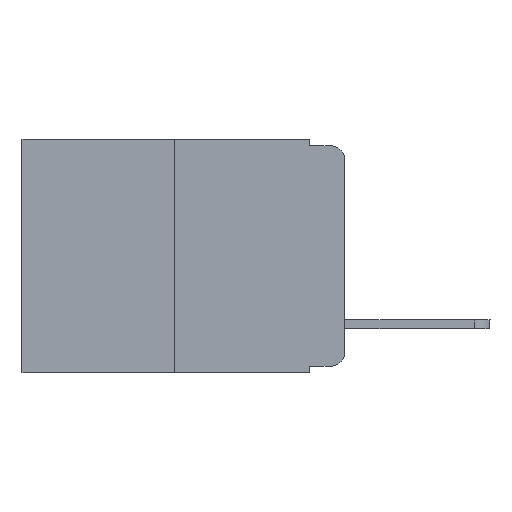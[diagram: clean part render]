
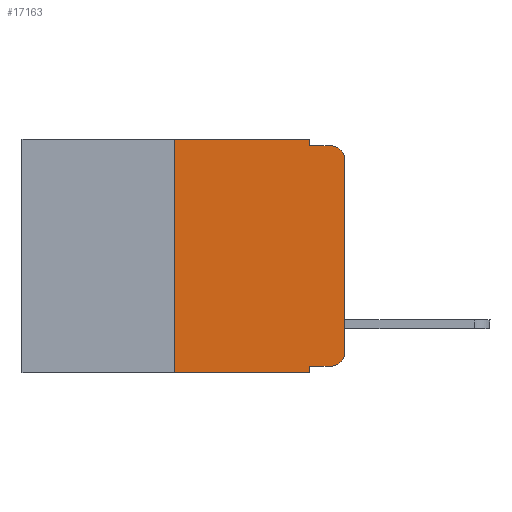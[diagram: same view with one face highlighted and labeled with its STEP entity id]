
A CAD part, left-side view. The second image highlights one B-rep face of the part: STEP entity #17163.
In plain terms, the highlighted planar face has unit normal (-1, 0, 0).
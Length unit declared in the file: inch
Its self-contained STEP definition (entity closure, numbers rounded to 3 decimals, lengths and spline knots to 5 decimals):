
#25 = CARTESIAN_POINT ( 'NONE',  ( 0., 0.473, 0. ) ) ;
#156 = LINE ( 'NONE', #4630, #2703 ) ;
#206 = EDGE_CURVE ( 'NONE', #1148, #16607, #7201, .T. ) ;
#306 = VECTOR ( 'NONE', #5939, 39.37008 ) ;
#526 = EDGE_CURVE ( 'NONE', #20060, #1148, #8143, .T. ) ;
#609 = LINE ( 'NONE', #7110, #16516 ) ;
#885 = EDGE_CURVE ( 'NONE', #12155, #20060, #12541, .T. ) ;
#1148 = VERTEX_POINT ( 'NONE', #8923 ) ;
#1955 = VECTOR ( 'NONE', #15496, 39.37008 ) ;
#2307 = CARTESIAN_POINT ( 'NONE',  ( 0., 0.02, -0.01 ) ) ;
#2349 = EDGE_CURVE ( 'NONE', #11535, #4945, #4373, .T. ) ;
#2442 = CARTESIAN_POINT ( 'NONE',  ( 0., 0.02, -0.333 ) ) ;
#2703 = VECTOR ( 'NONE', #9926, 39.37008 ) ;
#3430 = ORIENTED_EDGE ( 'NONE', *, *, #206, .T. ) ;
#3432 = DIRECTION ( 'NONE',  ( 0., 0., -1. ) ) ;
#3862 = CARTESIAN_POINT ( 'NONE',  ( 0., 0.473, -0.343 ) ) ;
#3900 = DIRECTION ( 'NONE',  ( 0., 0., -1. ) ) ;
#3972 = VERTEX_POINT ( 'NONE', #5733 ) ;
#4373 = LINE ( 'NONE', #19002, #14022 ) ;
#4630 = CARTESIAN_POINT ( 'NONE',  ( 0., 0.051, 0. ) ) ;
#4945 = VERTEX_POINT ( 'NONE', #18757 ) ;
#5733 = CARTESIAN_POINT ( 'NONE',  ( 0., 0.051, -0.01 ) ) ;
#5939 = DIRECTION ( 'NONE',  ( 0., -1., 0. ) ) ;
#6059 = VECTOR ( 'NONE', #16985, 39.37008 ) ;
#6770 = AXIS2_PLACEMENT_3D ( 'NONE', #25, #14555, #3432 ) ;
#7110 = CARTESIAN_POINT ( 'NONE',  ( 0., 0.473, 0. ) ) ;
#7201 = CIRCLE ( 'NONE', #10912, 0.02 ) ;
#7504 = CARTESIAN_POINT ( 'NONE',  ( 0., 0.051, 0. ) ) ;
#8056 = ORIENTED_EDGE ( 'NONE', *, *, #17466, .F. ) ;
#8143 = LINE ( 'NONE', #17993, #16339 ) ;
#8671 = ORIENTED_EDGE ( 'NONE', *, *, #885, .T. ) ;
#8803 = EDGE_CURVE ( 'NONE', #10711, #9276, #16306, .T. ) ;
#8923 = CARTESIAN_POINT ( 'NONE',  ( 0., 0., -0.03 ) ) ;
#8993 = ORIENTED_EDGE ( 'NONE', *, *, #526, .T. ) ;
#9030 = LINE ( 'NONE', #3862, #1955 ) ;
#9276 = VERTEX_POINT ( 'NONE', #16469 ) ;
#9844 = DIRECTION ( 'NONE',  ( 0., 0., -1. ) ) ;
#9926 = DIRECTION ( 'NONE',  ( 0., 0., -1. ) ) ;
#10392 = CARTESIAN_POINT ( 'NONE',  ( 0., 0.051, -0.333 ) ) ;
#10711 = VERTEX_POINT ( 'NONE', #15401 ) ;
#10912 = AXIS2_PLACEMENT_3D ( 'NONE', #11940, #11845, #3900 ) ;
#11369 = FACE_OUTER_BOUND ( 'NONE', #12561, .T. ) ;
#11535 = VERTEX_POINT ( 'NONE', #16652 ) ;
#11582 = PLANE ( 'NONE',  #6770 ) ;
#11619 = EDGE_CURVE ( 'NONE', #4945, #18305, #609, .T. ) ;
#11752 = ORIENTED_EDGE ( 'NONE', *, *, #2349, .F. ) ;
#11845 = DIRECTION ( 'NONE',  ( -1., 0., 0. ) ) ;
#11940 = CARTESIAN_POINT ( 'NONE',  ( 0., 0.02, -0.03 ) ) ;
#12155 = VERTEX_POINT ( 'NONE', #2442 ) ;
#12209 = LINE ( 'NONE', #10392, #6059 ) ;
#12312 = DIRECTION ( 'NONE',  ( 0., 0., 1. ) ) ;
#12541 = CIRCLE ( 'NONE', #16273, 0.02 ) ;
#12561 = EDGE_LOOP ( 'NONE', ( #8993, #3430, #8056, #15671, #16234, #11752, #13490, #19317, #12961, #8671 ) ) ;
#12621 = LINE ( 'NONE', #20562, #306 ) ;
#12871 = CARTESIAN_POINT ( 'NONE',  ( 0., 0., -0.313 ) ) ;
#12961 = ORIENTED_EDGE ( 'NONE', *, *, #17292, .T. ) ;
#13490 = ORIENTED_EDGE ( 'NONE', *, *, #16862, .T. ) ;
#13568 = DIRECTION ( 'NONE',  ( 0., -1., 0. ) ) ;
#14022 = VECTOR ( 'NONE', #12312, 39.37008 ) ;
#14555 = DIRECTION ( 'NONE',  ( 1., 0., 0. ) ) ;
#14594 = DIRECTION ( 'NONE',  ( 0., 0., 1. ) ) ;
#14604 = CARTESIAN_POINT ( 'NONE',  ( 0., 0.051, 0. ) ) ;
#15401 = CARTESIAN_POINT ( 'NONE',  ( 0., 0.051, -0.333 ) ) ;
#15496 = DIRECTION ( 'NONE',  ( 0., -1., 0. ) ) ;
#15671 = ORIENTED_EDGE ( 'NONE', *, *, #19745, .F. ) ;
#16234 = ORIENTED_EDGE ( 'NONE', *, *, #11619, .F. ) ;
#16264 = CARTESIAN_POINT ( 'NONE',  ( 0., 0.02, -0.313 ) ) ;
#16273 = AXIS2_PLACEMENT_3D ( 'NONE', #16264, #17747, #20921 ) ;
#16306 = LINE ( 'NONE', #14604, #19289 ) ;
#16339 = VECTOR ( 'NONE', #14594, 39.37008 ) ;
#16469 = CARTESIAN_POINT ( 'NONE',  ( 0., 0.051, -0.343 ) ) ;
#16516 = VECTOR ( 'NONE', #13568, 39.37008 ) ;
#16607 = VERTEX_POINT ( 'NONE', #2307 ) ;
#16652 = CARTESIAN_POINT ( 'NONE',  ( 0., 0.25, -0.343 ) ) ;
#16862 = EDGE_CURVE ( 'NONE', #11535, #9276, #9030, .T. ) ;
#16985 = DIRECTION ( 'NONE',  ( 0., -1., 0. ) ) ;
#17163 = ADVANCED_FACE ( 'NONE', ( #11369 ), #11582, .F. ) ;
#17292 = EDGE_CURVE ( 'NONE', #10711, #12155, #12209, .T. ) ;
#17466 = EDGE_CURVE ( 'NONE', #3972, #16607, #12621, .T. ) ;
#17747 = DIRECTION ( 'NONE',  ( -1., 0., 0. ) ) ;
#17993 = CARTESIAN_POINT ( 'NONE',  ( 0., 0., 0. ) ) ;
#18305 = VERTEX_POINT ( 'NONE', #7504 ) ;
#18757 = CARTESIAN_POINT ( 'NONE',  ( 0., 0.25, 0. ) ) ;
#19002 = CARTESIAN_POINT ( 'NONE',  ( 0., 0.25, 0. ) ) ;
#19289 = VECTOR ( 'NONE', #9844, 39.37008 ) ;
#19317 = ORIENTED_EDGE ( 'NONE', *, *, #8803, .F. ) ;
#19745 = EDGE_CURVE ( 'NONE', #18305, #3972, #156, .T. ) ;
#20060 = VERTEX_POINT ( 'NONE', #12871 ) ;
#20562 = CARTESIAN_POINT ( 'NONE',  ( 0., 0.051, -0.01 ) ) ;
#20921 = DIRECTION ( 'NONE',  ( 0., 0., -1. ) ) ;
